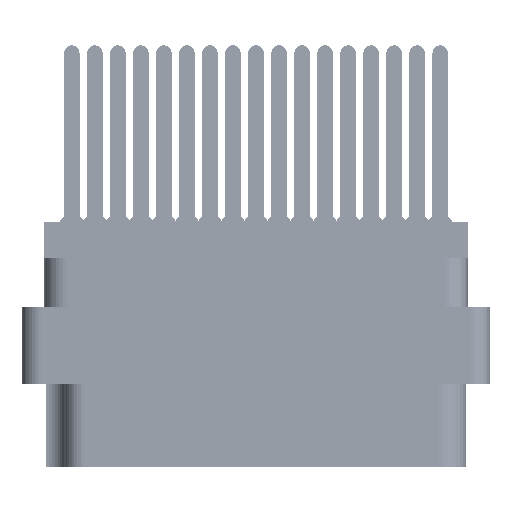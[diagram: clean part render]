
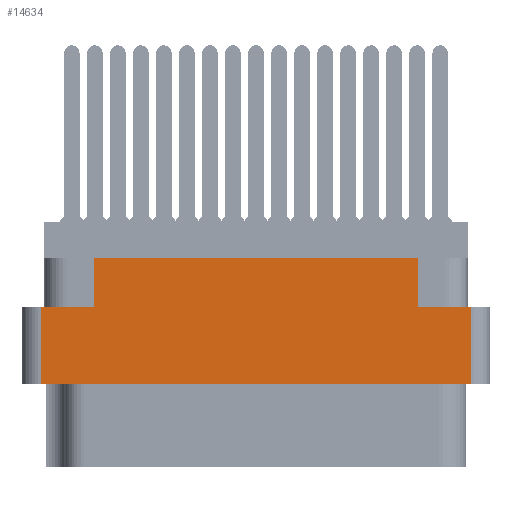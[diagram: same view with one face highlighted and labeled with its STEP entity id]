
A CAD part, left-side view. The second image highlights one B-rep face of the part: STEP entity #14634.
In plain terms, the highlighted planar face has unit normal (-1, 0, 0).
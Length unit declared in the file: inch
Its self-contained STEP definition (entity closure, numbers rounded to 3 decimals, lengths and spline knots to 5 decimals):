
#5 = CARTESIAN_POINT ( 'NONE',  ( -1.375, 0.5285, -0.117 ) ) ;
#3138 = CARTESIAN_POINT ( 'NONE',  ( -1.375, -0.7625, -0.798 ) ) ;
#3413 = VECTOR ( 'NONE', #70197, 39.37008 ) ;
#4117 = CARTESIAN_POINT ( 'NONE',  ( -1.375, 0.5285, -0.277 ) ) ;
#7029 = VERTEX_POINT ( 'NONE', #63048 ) ;
#8828 = DIRECTION ( 'NONE',  ( 0., 0., 1. ) ) ;
#8965 = ORIENTED_EDGE ( 'NONE', *, *, #79741, .F. ) ;
#13056 = VECTOR ( 'NONE', #8828, 39.37008 ) ;
#13552 = DIRECTION ( 'NONE',  ( 0., -1., 0. ) ) ;
#13936 = ORIENTED_EDGE ( 'NONE', *, *, #71568, .T. ) ;
#14262 = VERTEX_POINT ( 'NONE', #5 ) ;
#14634 = ADVANCED_FACE ( 'NONE', ( #48985 ), #39431, .T. ) ;
#16240 = VECTOR ( 'NONE', #18201, 39.37008 ) ;
#18201 = DIRECTION ( 'NONE',  ( 0., 0., 1. ) ) ;
#18554 = EDGE_CURVE ( 'NONE', #7029, #14262, #35595, .T. ) ;
#19211 = CARTESIAN_POINT ( 'NONE',  ( -1.375, -0.7005, -0.277 ) ) ;
#20400 = CARTESIAN_POINT ( 'NONE',  ( -1.375, -0.5285, -0.117 ) ) ;
#20911 = LINE ( 'NONE', #72372, #50436 ) ;
#21529 = LINE ( 'NONE', #71147, #44219 ) ;
#22242 = VECTOR ( 'NONE', #32147, 39.37008 ) ;
#32039 = VERTEX_POINT ( 'NONE', #94210 ) ;
#32147 = DIRECTION ( 'NONE',  ( 0., 1., 0. ) ) ;
#32754 = CARTESIAN_POINT ( 'NONE',  ( -1.375, -0.7005, -0.529 ) ) ;
#35209 = CARTESIAN_POINT ( 'NONE',  ( -1.375, 0.7005, -0.277 ) ) ;
#35595 = LINE ( 'NONE', #4117, #16240 ) ;
#37523 = EDGE_CURVE ( 'NONE', #32039, #55293, #21529, .T. ) ;
#39431 = PLANE ( 'NONE',  #63079 ) ;
#40627 = ORIENTED_EDGE ( 'NONE', *, *, #37523, .F. ) ;
#41186 = EDGE_CURVE ( 'NONE', #14262, #47609, #20911, .T. ) ;
#41550 = LINE ( 'NONE', #75572, #22242 ) ;
#42017 = VECTOR ( 'NONE', #53936, 39.37008 ) ;
#44219 = VECTOR ( 'NONE', #57462, 39.37008 ) ;
#46691 = LINE ( 'NONE', #62251, #3413 ) ;
#47609 = VERTEX_POINT ( 'NONE', #20400 ) ;
#48985 = FACE_OUTER_BOUND ( 'NONE', #93092, .T. ) ;
#50436 = VECTOR ( 'NONE', #13552, 39.37008 ) ;
#51770 = CARTESIAN_POINT ( 'NONE',  ( -1.375, -0.5285, -0.277 ) ) ;
#53936 = DIRECTION ( 'NONE',  ( 0., -1., 0. ) ) ;
#54032 = DIRECTION ( 'NONE',  ( 0., 0., 1. ) ) ;
#54328 = DIRECTION ( 'NONE',  ( -1., 0., 0. ) ) ;
#54661 = EDGE_CURVE ( 'NONE', #66127, #7029, #89839, .T. ) ;
#55293 = VERTEX_POINT ( 'NONE', #19211 ) ;
#57328 = LINE ( 'NONE', #61101, #81159 ) ;
#57462 = DIRECTION ( 'NONE',  ( 0., -1., 0. ) ) ;
#59414 = EDGE_CURVE ( 'NONE', #66127, #73970, #46691, .T. ) ;
#60829 = ORIENTED_EDGE ( 'NONE', *, *, #18554, .F. ) ;
#61101 = CARTESIAN_POINT ( 'NONE',  ( -1.375, -0.7005, -0.798 ) ) ;
#62251 = CARTESIAN_POINT ( 'NONE',  ( -1.375, 0.7005, -0.798 ) ) ;
#63048 = CARTESIAN_POINT ( 'NONE',  ( -1.375, 0.5285, -0.277 ) ) ;
#63079 = AXIS2_PLACEMENT_3D ( 'NONE', #3138, #54328, #54032 ) ;
#63157 = ORIENTED_EDGE ( 'NONE', *, *, #54661, .F. ) ;
#66127 = VERTEX_POINT ( 'NONE', #35209 ) ;
#69909 = LINE ( 'NONE', #51770, #13056 ) ;
#70197 = DIRECTION ( 'NONE',  ( 0., 0., -1. ) ) ;
#71147 = CARTESIAN_POINT ( 'NONE',  ( -1.375, 0., -0.277 ) ) ;
#71568 = EDGE_CURVE ( 'NONE', #74277, #55293, #57328, .T. ) ;
#72372 = CARTESIAN_POINT ( 'NONE',  ( -1.375, 0.7625, -0.117 ) ) ;
#73888 = ORIENTED_EDGE ( 'NONE', *, *, #86327, .T. ) ;
#73970 = VERTEX_POINT ( 'NONE', #87323 ) ;
#74277 = VERTEX_POINT ( 'NONE', #32754 ) ;
#75572 = CARTESIAN_POINT ( 'NONE',  ( -1.375, 0., -0.529 ) ) ;
#76302 = DIRECTION ( 'NONE',  ( 0., 0., 1. ) ) ;
#77243 = ORIENTED_EDGE ( 'NONE', *, *, #41186, .F. ) ;
#77700 = ORIENTED_EDGE ( 'NONE', *, *, #59414, .T. ) ;
#79741 = EDGE_CURVE ( 'NONE', #74277, #73970, #41550, .T. ) ;
#81159 = VECTOR ( 'NONE', #76302, 39.37008 ) ;
#86327 = EDGE_CURVE ( 'NONE', #32039, #47609, #69909, .T. ) ;
#87323 = CARTESIAN_POINT ( 'NONE',  ( -1.375, 0.7005, -0.529 ) ) ;
#89839 = LINE ( 'NONE', #90086, #42017 ) ;
#90086 = CARTESIAN_POINT ( 'NONE',  ( -1.375, 0., -0.277 ) ) ;
#93092 = EDGE_LOOP ( 'NONE', ( #63157, #77700, #8965, #13936, #40627, #73888, #77243, #60829 ) ) ;
#94210 = CARTESIAN_POINT ( 'NONE',  ( -1.375, -0.5285, -0.277 ) ) ;
